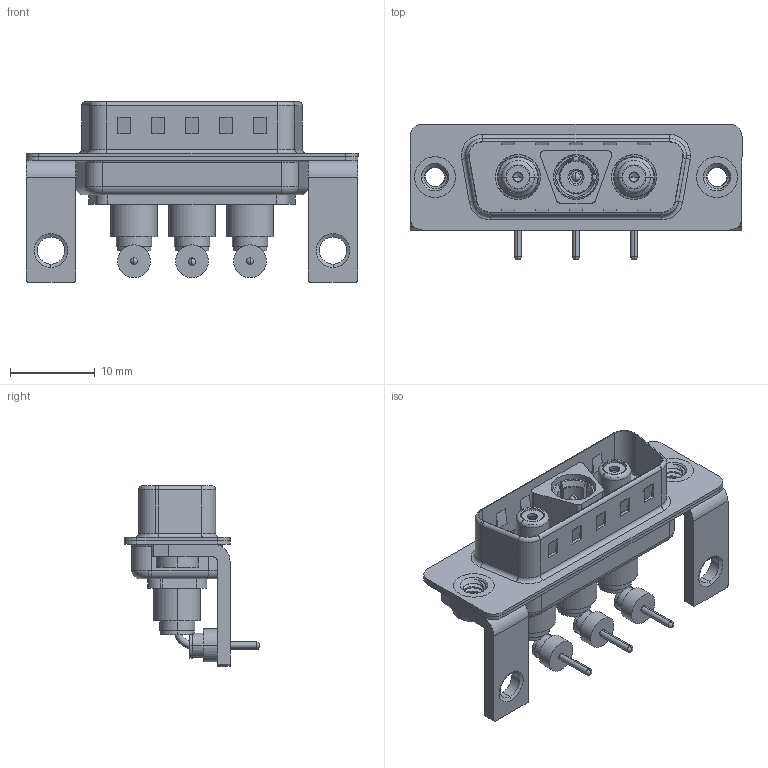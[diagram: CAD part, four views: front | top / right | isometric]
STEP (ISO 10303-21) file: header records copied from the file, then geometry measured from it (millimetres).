
FILE_DESCRIPTION (( 'STEP AP203' ), '1' );
FILE_NAME ('629-3WK3240-5NC.STEP', '2022-05-05T09:50:58', ( '' ), ( '' ), 'SwSTEP 2.0', 'SolidWorks 2020', '' );
FILE_SCHEMA (( 'CONFIG_CONTROL_DESIGN' ));
Length unit declared in the file: millimetre
Products named in the file (18): Co-Ax Jack_RA PC Tail; 629Combo Threaded Rivet_2; Insulator RA Pin; Co-Ax Plug_RA PC Tail; Co-Ax Jack Assy_RA; Locking Collar; 629Combo Stabilizer Bracket; 629Combo Shell Front_15 Contacts; Insulator Socket; 629Combo Housing_3WK3; Co-Ax Plug Assy_RA; 629-3WK3240-5NC; Socket_RA; Insulator Pin_Straight PC Tail; Pin_RA; 629Combo Shell Rear_15 Contacts; Insulator Socket 2
Assembly tree (27 placements, depth 3):
  629-3WK3240-5NC
    629Combo Housing_3WK3
    629Combo Shell Rear_15 Contacts
    629Combo Shell Front_15 Contacts
    629Combo Threaded Rivet_2  x2
    629Combo Stabilizer Bracket  x2
    Co-Ax Plug Assy_RA
      Co-Ax Plug_RA PC Tail
      Insulator Pin_Straight PC Tail
      Pin_RA
      Locking Collar
      Insulator RA Pin
    Co-Ax Jack Assy_RA
      Co-Ax Jack_RA PC Tail
      Insulator Socket
      Insulator Socket 2
      Locking Collar
      Socket_RA
      Insulator RA Pin
    Co-Ax Jack Assy_RA
      Co-Ax Jack_RA PC Tail
      Insulator Socket
      Insulator Socket 2
      Locking Collar
      Socket_RA
      Insulator RA Pin
Bounding box: 39.2 x 16 x 21.3 mm (x, y, z)
Volume: 2586.6 mm3; surface area: 7267.9 mm2
Topology: 24 solids, 24 shells, 765 faces, 1842 edges, 1164 vertices
Faces by surface type: cylinder 343, plane 276, torus 68, cone 61, bspline 9, sphere 8
Entity records: 20733 total; most frequent: CARTESIAN_POINT 4582, DIRECTION 3134, ORIENTED_EDGE 2778, EDGE_CURVE 1389, AXIS2_PLACEMENT_3D 1217, VERTEX_POINT 882, LINE 700, VECTOR 700
